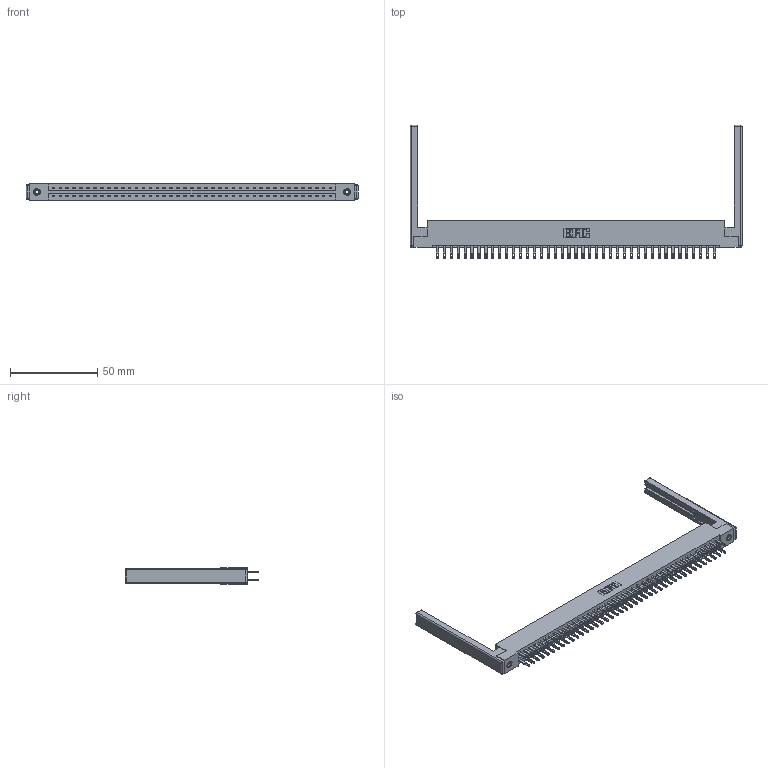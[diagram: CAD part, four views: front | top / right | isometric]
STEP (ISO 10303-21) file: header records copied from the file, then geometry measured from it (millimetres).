
FILE_DESCRIPTION (( 'STEP AP203' ), '1' );
FILE_NAME ('337-082-500-268.STEP', '2019-10-10T12:44:55', ( '' ), ( '' ), 'SwSTEP 2.0', 'SolidWorks 2016', '' );
FILE_SCHEMA (( 'CONFIG_CONTROL_DESIGN' ));
Length unit declared in the file: inch
Products named in the file (5): 345-292-001_345-293-100; 345-250-001_345-250-001-102; 337-082-500-268; 307-220-068; 337 Part_Flush Mounting Lugs - 0.156 Dia-TI
Assembly tree (87 placements, depth 2):
  337-082-500-268
    337 Part_Flush Mounting Lugs - 0.156 Dia-TI
    345-292-001_345-293-100  x82
    345-250-001_345-250-001-102  x2
    307-220-068  x2
Bounding box: 189.89 x 76.59 x 9.4 mm (x, y, z)
Volume: 24634.2 mm3; surface area: 27826.5 mm2
Topology: 87 solids, 87 shells, 4368 faces, 13247 edges, 8810 vertices
Faces by surface type: plane 2782, cylinder 1562, cone 12, sphere 8, torus 4
Entity records: 34608 total; most frequent: CARTESIAN_POINT 5795, ORIENTED_EDGE 5720, DIRECTION 5002, EDGE_CURVE 2860, LINE 2678, VECTOR 2678, VERTEX_POINT 1898, AXIS2_PLACEMENT_3D 1162
